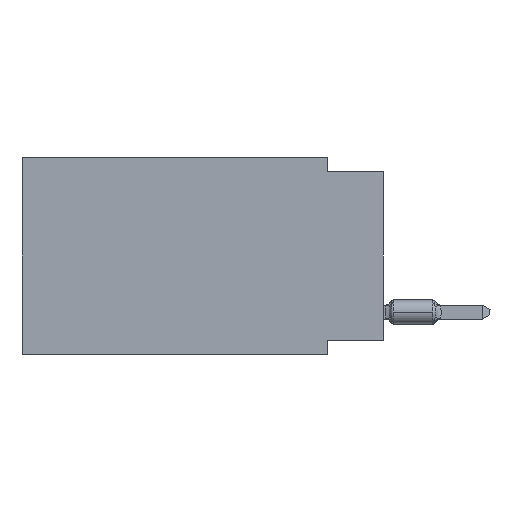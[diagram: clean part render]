
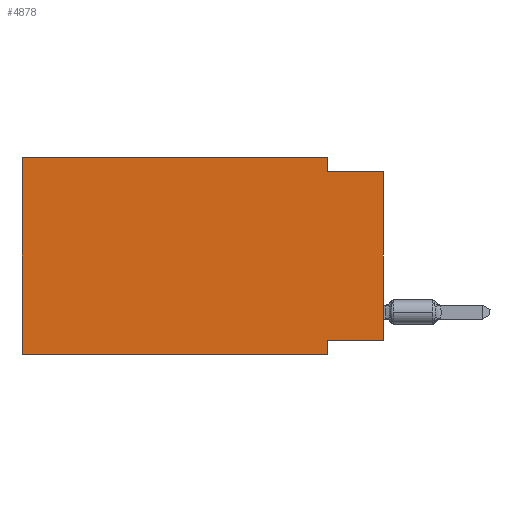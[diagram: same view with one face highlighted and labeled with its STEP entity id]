
A CAD part, left-side view. The second image highlights one B-rep face of the part: STEP entity #4878.
In plain terms, the highlighted planar face has unit normal (-1, 0, 0).
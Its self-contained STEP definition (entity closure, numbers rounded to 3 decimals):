
#467 = VECTOR ( 'NONE', #3998, 1000. ) ;
#764 = ORIENTED_EDGE ( 'NONE', *, *, #2737, .T. ) ;
#1277 = ORIENTED_EDGE ( 'NONE', *, *, #8560, .F. ) ;
#1397 = ORIENTED_EDGE ( 'NONE', *, *, #6237, .F. ) ;
#1871 = CARTESIAN_POINT ( 'NONE',  ( 0., 16.383, -8.89 ) ) ;
#2010 = ORIENTED_EDGE ( 'NONE', *, *, #4721, .F. ) ;
#2152 = DIRECTION ( 'NONE',  ( 0., 0., -1. ) ) ;
#2556 = VECTOR ( 'NONE', #4597, 1000. ) ;
#2737 = EDGE_CURVE ( 'NONE', #5863, #17359, #14414, .T. ) ;
#3320 = CARTESIAN_POINT ( 'NONE',  ( 0., 2.54, -8.89 ) ) ;
#3452 = EDGE_CURVE ( 'NONE', #16999, #18807, #4711, .T. ) ;
#3629 = CARTESIAN_POINT ( 'NONE',  ( 0., 16.383, 0. ) ) ;
#3691 = VECTOR ( 'NONE', #17238, 1000. ) ;
#3998 = DIRECTION ( 'NONE',  ( 0., 0., 1. ) ) ;
#4083 = VECTOR ( 'NONE', #15061, 1000. ) ;
#4220 = DIRECTION ( 'NONE',  ( 0., 0., -1. ) ) ;
#4500 = VERTEX_POINT ( 'NONE', #19252 ) ;
#4597 = DIRECTION ( 'NONE',  ( 0., -1., 0. ) ) ;
#4711 = LINE ( 'NONE', #3629, #3691 ) ;
#4721 = EDGE_CURVE ( 'NONE', #18807, #19571, #11085, .T. ) ;
#4878 = ADVANCED_FACE ( 'NONE', ( #19228 ), #7302, .F. ) ;
#5406 = CARTESIAN_POINT ( 'NONE',  ( 0., 16.383, 0. ) ) ;
#5799 = CARTESIAN_POINT ( 'NONE',  ( 0., 16.383, -8.89 ) ) ;
#5863 = VERTEX_POINT ( 'NONE', #10424 ) ;
#6185 = CARTESIAN_POINT ( 'NONE',  ( 0., 0., -0.635 ) ) ;
#6237 = EDGE_CURVE ( 'NONE', #14166, #16999, #11357, .T. ) ;
#6599 = DIRECTION ( 'NONE',  ( 0., 0., -1. ) ) ;
#7205 = LINE ( 'NONE', #5799, #2556 ) ;
#7302 = PLANE ( 'NONE',  #14704 ) ;
#7390 = DIRECTION ( 'NONE',  ( 1., 0., 0. ) ) ;
#7512 = VECTOR ( 'NONE', #15988, 1000. ) ;
#8547 = EDGE_CURVE ( 'NONE', #5863, #4500, #13678, .T. ) ;
#8560 = EDGE_CURVE ( 'NONE', #19571, #17359, #12175, .T. ) ;
#10424 = CARTESIAN_POINT ( 'NONE',  ( 0., 0., -8.255 ) ) ;
#10470 = CARTESIAN_POINT ( 'NONE',  ( 0., 16.383, 0. ) ) ;
#10696 = CARTESIAN_POINT ( 'NONE',  ( 0., 2.54, 0. ) ) ;
#10973 = DIRECTION ( 'NONE',  ( 0., 1., 0. ) ) ;
#11085 = LINE ( 'NONE', #11284, #13559 ) ;
#11284 = CARTESIAN_POINT ( 'NONE',  ( 0., 2.54, 0. ) ) ;
#11357 = LINE ( 'NONE', #17215, #467 ) ;
#11397 = EDGE_CURVE ( 'NONE', #4500, #15086, #14066, .T. ) ;
#11583 = VECTOR ( 'NONE', #6599, 1000. ) ;
#11926 = ORIENTED_EDGE ( 'NONE', *, *, #19209, .T. ) ;
#12175 = LINE ( 'NONE', #18452, #4083 ) ;
#12340 = ORIENTED_EDGE ( 'NONE', *, *, #8547, .F. ) ;
#12376 = CARTESIAN_POINT ( 'NONE',  ( 0., 0., -8.255 ) ) ;
#12754 = ORIENTED_EDGE ( 'NONE', *, *, #11397, .F. ) ;
#13559 = VECTOR ( 'NONE', #2152, 1000. ) ;
#13678 = LINE ( 'NONE', #12376, #17397 ) ;
#14014 = EDGE_LOOP ( 'NONE', ( #764, #1277, #2010, #15704, #1397, #11926, #12754, #12340 ) ) ;
#14066 = LINE ( 'NONE', #3320, #11583 ) ;
#14166 = VERTEX_POINT ( 'NONE', #1871 ) ;
#14414 = LINE ( 'NONE', #19177, #7512 ) ;
#14523 = CARTESIAN_POINT ( 'NONE',  ( 0., 2.54, -8.89 ) ) ;
#14704 = AXIS2_PLACEMENT_3D ( 'NONE', #10470, #7390, #4220 ) ;
#15061 = DIRECTION ( 'NONE',  ( 0., -1., 0. ) ) ;
#15086 = VERTEX_POINT ( 'NONE', #14523 ) ;
#15704 = ORIENTED_EDGE ( 'NONE', *, *, #3452, .F. ) ;
#15988 = DIRECTION ( 'NONE',  ( 0., 0., 1. ) ) ;
#16999 = VERTEX_POINT ( 'NONE', #5406 ) ;
#17215 = CARTESIAN_POINT ( 'NONE',  ( 0., 16.383, 0. ) ) ;
#17238 = DIRECTION ( 'NONE',  ( 0., -1., 0. ) ) ;
#17359 = VERTEX_POINT ( 'NONE', #6185 ) ;
#17397 = VECTOR ( 'NONE', #10973, 1000. ) ;
#18452 = CARTESIAN_POINT ( 'NONE',  ( 0., 0., -0.635 ) ) ;
#18807 = VERTEX_POINT ( 'NONE', #10696 ) ;
#19031 = CARTESIAN_POINT ( 'NONE',  ( 0., 2.54, -0.635 ) ) ;
#19177 = CARTESIAN_POINT ( 'NONE',  ( 0., 0., 0. ) ) ;
#19209 = EDGE_CURVE ( 'NONE', #14166, #15086, #7205, .T. ) ;
#19228 = FACE_OUTER_BOUND ( 'NONE', #14014, .T. ) ;
#19252 = CARTESIAN_POINT ( 'NONE',  ( 0., 2.54, -8.255 ) ) ;
#19571 = VERTEX_POINT ( 'NONE', #19031 ) ;
